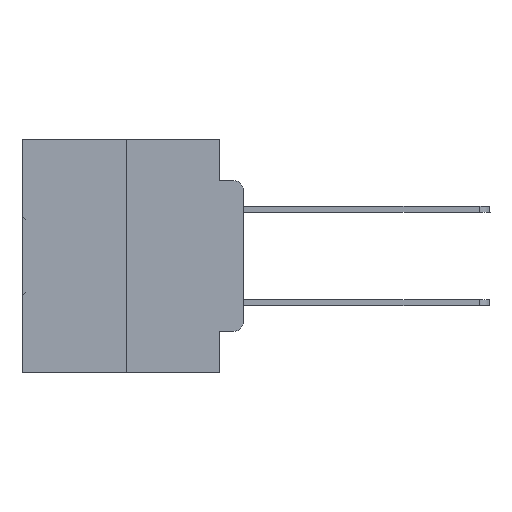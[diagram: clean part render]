
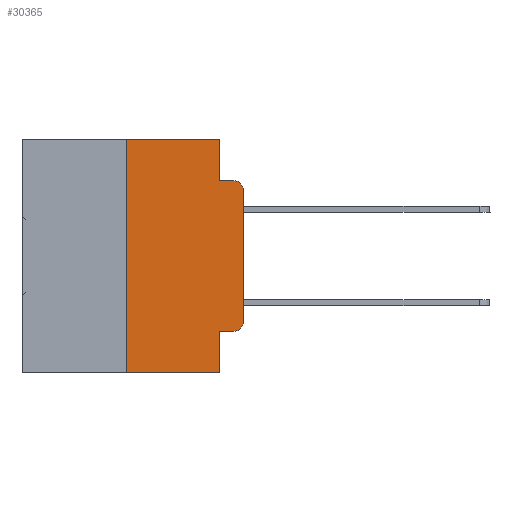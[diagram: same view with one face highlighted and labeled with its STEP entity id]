
A CAD part, left-side view. The second image highlights one B-rep face of the part: STEP entity #30365.
In plain terms, the highlighted planar face has unit normal (-1, 0, 0).
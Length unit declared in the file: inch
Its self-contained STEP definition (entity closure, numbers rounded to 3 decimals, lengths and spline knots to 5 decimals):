
#546 = CARTESIAN_POINT ( 'NONE',  ( 0., 0.051, -0.0885 ) ) ;
#1926 = CARTESIAN_POINT ( 'NONE',  ( 0., 0.473, -0.5 ) ) ;
#2457 = FACE_OUTER_BOUND ( 'NONE', #20874, .T. ) ;
#2605 = LINE ( 'NONE', #25988, #31486 ) ;
#2635 = ORIENTED_EDGE ( 'NONE', *, *, #6074, .T. ) ;
#3161 = DIRECTION ( 'NONE',  ( 1., 0., 0. ) ) ;
#3265 = CARTESIAN_POINT ( 'NONE',  ( 0., 0.051, -0.0885 ) ) ;
#3401 = CARTESIAN_POINT ( 'NONE',  ( 0., 0.051, 0. ) ) ;
#4799 = LINE ( 'NONE', #546, #23151 ) ;
#5481 = CARTESIAN_POINT ( 'NONE',  ( 0., 0.25, -0.5 ) ) ;
#6031 = LINE ( 'NONE', #28092, #7340 ) ;
#6074 = EDGE_CURVE ( 'NONE', #7074, #35152, #33989, .T. ) ;
#6260 = DIRECTION ( 'NONE',  ( 0., -1., 0. ) ) ;
#6427 = ORIENTED_EDGE ( 'NONE', *, *, #17468, .T. ) ;
#6774 = VECTOR ( 'NONE', #26871, 39.37008 ) ;
#6947 = CARTESIAN_POINT ( 'NONE',  ( 0., 0.02, -0.1085 ) ) ;
#7074 = VERTEX_POINT ( 'NONE', #22677 ) ;
#7283 = VECTOR ( 'NONE', #17810, 39.37008 ) ;
#7289 = EDGE_CURVE ( 'NONE', #8009, #8282, #22867, .T. ) ;
#7340 = VECTOR ( 'NONE', #31405, 39.37008 ) ;
#7556 = ORIENTED_EDGE ( 'NONE', *, *, #34582, .F. ) ;
#8009 = VERTEX_POINT ( 'NONE', #24334 ) ;
#8282 = VERTEX_POINT ( 'NONE', #3401 ) ;
#8300 = VERTEX_POINT ( 'NONE', #25666 ) ;
#9204 = CARTESIAN_POINT ( 'NONE',  ( 0., 0.051, 0. ) ) ;
#9224 = CARTESIAN_POINT ( 'NONE',  ( 0., 0., -0.1085 ) ) ;
#9943 = AXIS2_PLACEMENT_3D ( 'NONE', #23712, #28709, #11979 ) ;
#10644 = ORIENTED_EDGE ( 'NONE', *, *, #29771, .F. ) ;
#10746 = LINE ( 'NONE', #9204, #7283 ) ;
#11586 = PLANE ( 'NONE',  #13703 ) ;
#11957 = VECTOR ( 'NONE', #6260, 39.37008 ) ;
#11979 = DIRECTION ( 'NONE',  ( 0., 0., -1. ) ) ;
#12922 = DIRECTION ( 'NONE',  ( 0., 0., -1. ) ) ;
#13671 = VECTOR ( 'NONE', #26080, 39.37008 ) ;
#13693 = VERTEX_POINT ( 'NONE', #18545 ) ;
#13703 = AXIS2_PLACEMENT_3D ( 'NONE', #17155, #3161, #25793 ) ;
#14184 = LINE ( 'NONE', #1926, #6774 ) ;
#17155 = CARTESIAN_POINT ( 'NONE',  ( 0., 0.473, 0. ) ) ;
#17317 = AXIS2_PLACEMENT_3D ( 'NONE', #6947, #18260, #12922 ) ;
#17468 = EDGE_CURVE ( 'NONE', #35152, #8300, #27010, .T. ) ;
#17810 = DIRECTION ( 'NONE',  ( 0., 0., -1. ) ) ;
#17834 = VERTEX_POINT ( 'NONE', #5481 ) ;
#18044 = VERTEX_POINT ( 'NONE', #3265 ) ;
#18260 = DIRECTION ( 'NONE',  ( -1., 0., 0. ) ) ;
#18545 = CARTESIAN_POINT ( 'NONE',  ( 0., 0.02, -0.0885 ) ) ;
#19021 = VECTOR ( 'NONE', #21084, 39.37008 ) ;
#20057 = DIRECTION ( 'NONE',  ( 0., -1., 0. ) ) ;
#20874 = EDGE_LOOP ( 'NONE', ( #23224, #26355, #33757, #10644, #34826, #31781, #30632, #7556, #2635, #6427 ) ) ;
#21084 = DIRECTION ( 'NONE',  ( 0., -1., 0. ) ) ;
#21208 = CARTESIAN_POINT ( 'NONE',  ( 0., 0.051, -0.4115 ) ) ;
#22380 = CARTESIAN_POINT ( 'NONE',  ( 0., 0.051, -0.5 ) ) ;
#22677 = CARTESIAN_POINT ( 'NONE',  ( 0., 0.051, -0.4115 ) ) ;
#22867 = LINE ( 'NONE', #28486, #11957 ) ;
#23151 = VECTOR ( 'NONE', #20057, 39.37008 ) ;
#23224 = ORIENTED_EDGE ( 'NONE', *, *, #23969, .T. ) ;
#23712 = CARTESIAN_POINT ( 'NONE',  ( 0., 0.02, -0.3915 ) ) ;
#23969 = EDGE_CURVE ( 'NONE', #8300, #24528, #6031, .T. ) ;
#24334 = CARTESIAN_POINT ( 'NONE',  ( 0., 0.25, 0. ) ) ;
#24528 = VERTEX_POINT ( 'NONE', #9224 ) ;
#25666 = CARTESIAN_POINT ( 'NONE',  ( 0., 0., -0.3915 ) ) ;
#25793 = DIRECTION ( 'NONE',  ( 0., 0., -1. ) ) ;
#25988 = CARTESIAN_POINT ( 'NONE',  ( 0., 0.051, 0. ) ) ;
#26080 = DIRECTION ( 'NONE',  ( 0., 0., 1. ) ) ;
#26313 = CARTESIAN_POINT ( 'NONE',  ( 0., 0.25, 0. ) ) ;
#26355 = ORIENTED_EDGE ( 'NONE', *, *, #35528, .T. ) ;
#26546 = EDGE_CURVE ( 'NONE', #17834, #31441, #14184, .T. ) ;
#26871 = DIRECTION ( 'NONE',  ( 0., -1., 0. ) ) ;
#27010 = CIRCLE ( 'NONE', #9943, 0.02 ) ;
#27585 = EDGE_CURVE ( 'NONE', #17834, #8009, #36003, .T. ) ;
#27642 = CARTESIAN_POINT ( 'NONE',  ( 0., 0.02, -0.4115 ) ) ;
#28092 = CARTESIAN_POINT ( 'NONE',  ( 0., 0., 0. ) ) ;
#28486 = CARTESIAN_POINT ( 'NONE',  ( 0., 0.473, 0. ) ) ;
#28709 = DIRECTION ( 'NONE',  ( -1., 0., 0. ) ) ;
#29771 = EDGE_CURVE ( 'NONE', #8282, #18044, #10746, .T. ) ;
#30365 = ADVANCED_FACE ( 'NONE', ( #2457 ), #11586, .F. ) ;
#30632 = ORIENTED_EDGE ( 'NONE', *, *, #26546, .T. ) ;
#31405 = DIRECTION ( 'NONE',  ( 0., 0., 1. ) ) ;
#31441 = VERTEX_POINT ( 'NONE', #22380 ) ;
#31486 = VECTOR ( 'NONE', #31745, 39.37008 ) ;
#31745 = DIRECTION ( 'NONE',  ( 0., 0., -1. ) ) ;
#31781 = ORIENTED_EDGE ( 'NONE', *, *, #27585, .F. ) ;
#31874 = CIRCLE ( 'NONE', #17317, 0.02 ) ;
#33757 = ORIENTED_EDGE ( 'NONE', *, *, #34483, .F. ) ;
#33989 = LINE ( 'NONE', #21208, #19021 ) ;
#34483 = EDGE_CURVE ( 'NONE', #18044, #13693, #4799, .T. ) ;
#34582 = EDGE_CURVE ( 'NONE', #7074, #31441, #2605, .T. ) ;
#34826 = ORIENTED_EDGE ( 'NONE', *, *, #7289, .F. ) ;
#35152 = VERTEX_POINT ( 'NONE', #27642 ) ;
#35528 = EDGE_CURVE ( 'NONE', #24528, #13693, #31874, .T. ) ;
#36003 = LINE ( 'NONE', #26313, #13671 ) ;
